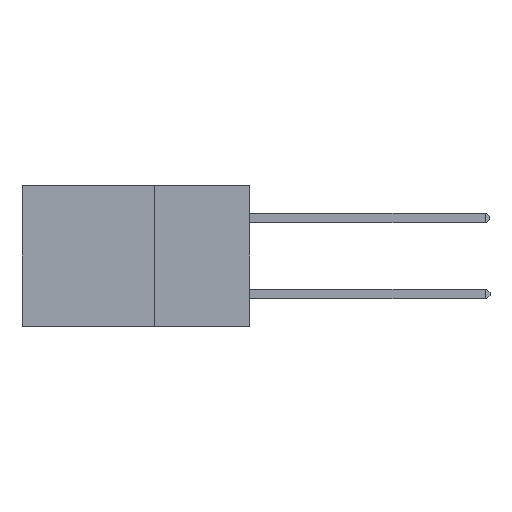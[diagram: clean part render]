
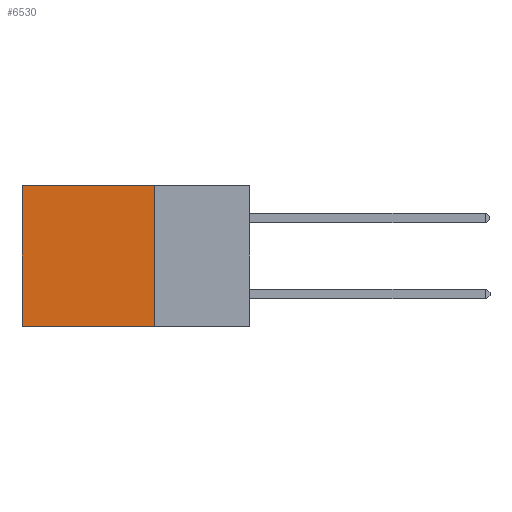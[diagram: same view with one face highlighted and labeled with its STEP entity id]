
A CAD part, left-side view. The second image highlights one B-rep face of the part: STEP entity #6530.
In plain terms, the highlighted planar face has unit normal (-1, 0, 0).
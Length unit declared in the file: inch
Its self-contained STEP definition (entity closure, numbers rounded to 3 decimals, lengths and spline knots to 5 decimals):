
#304 = AXIS2_PLACEMENT_3D ( 'NONE', #11808, #3369, #13177 ) ;
#1356 = EDGE_CURVE ( 'NONE', #13625, #13958, #12016, .T. ) ;
#2457 = CARTESIAN_POINT ( 'NONE',  ( 0.2875, 0.6, 0. ) ) ;
#3369 = DIRECTION ( 'NONE',  ( 1., 0., 0. ) ) ;
#3819 = EDGE_CURVE ( 'NONE', #12779, #13625, #6943, .T. ) ;
#3874 = EDGE_CURVE ( 'NONE', #12779, #17033, #13856, .T. ) ;
#5580 = EDGE_CURVE ( 'NONE', #17033, #13958, #14398, .T. ) ;
#6530 = ADVANCED_FACE ( 'NONE', ( #17355 ), #17137, .F. ) ;
#6943 = LINE ( 'NONE', #14657, #17375 ) ;
#7065 = VECTOR ( 'NONE', #17627, 39.37008 ) ;
#8341 = VECTOR ( 'NONE', #17480, 39.37008 ) ;
#11509 = EDGE_LOOP ( 'NONE', ( #13700, #13780, #13813, #13905 ) ) ;
#11808 = CARTESIAN_POINT ( 'NONE',  ( 0.2875, 0.25, 0. ) ) ;
#12016 = LINE ( 'NONE', #17886, #8341 ) ;
#12779 = VERTEX_POINT ( 'NONE', #16574 ) ;
#13177 = DIRECTION ( 'NONE',  ( 0., 0., -1. ) ) ;
#13539 = CARTESIAN_POINT ( 'NONE',  ( 0.2875, 0.6, 0. ) ) ;
#13625 = VERTEX_POINT ( 'NONE', #15833 ) ;
#13700 = ORIENTED_EDGE ( 'NONE', *, *, #5580, .T. ) ;
#13766 = DIRECTION ( 'NONE',  ( 0., 1., 0. ) ) ;
#13780 = ORIENTED_EDGE ( 'NONE', *, *, #1356, .F. ) ;
#13813 = ORIENTED_EDGE ( 'NONE', *, *, #3819, .F. ) ;
#13856 = LINE ( 'NONE', #13875, #16576 ) ;
#13875 = CARTESIAN_POINT ( 'NONE',  ( 0.2875, 0.25, 0. ) ) ;
#13905 = ORIENTED_EDGE ( 'NONE', *, *, #3874, .T. ) ;
#13958 = VERTEX_POINT ( 'NONE', #15017 ) ;
#14398 = LINE ( 'NONE', #2457, #7065 ) ;
#14534 = DIRECTION ( 'NONE',  ( 0., 0., -1. ) ) ;
#14657 = CARTESIAN_POINT ( 'NONE',  ( 0.2875, 0.25, 0. ) ) ;
#15017 = CARTESIAN_POINT ( 'NONE',  ( 0.2875, 0.6, -0.37 ) ) ;
#15833 = CARTESIAN_POINT ( 'NONE',  ( 0.2875, 0.25, -0.37 ) ) ;
#16574 = CARTESIAN_POINT ( 'NONE',  ( 0.2875, 0.25, 0. ) ) ;
#16576 = VECTOR ( 'NONE', #13766, 39.37008 ) ;
#17033 = VERTEX_POINT ( 'NONE', #13539 ) ;
#17137 = PLANE ( 'NONE',  #304 ) ;
#17355 = FACE_OUTER_BOUND ( 'NONE', #11509, .T. ) ;
#17375 = VECTOR ( 'NONE', #14534, 39.37008 ) ;
#17480 = DIRECTION ( 'NONE',  ( 0., 1., 0. ) ) ;
#17627 = DIRECTION ( 'NONE',  ( 0., 0., -1. ) ) ;
#17886 = CARTESIAN_POINT ( 'NONE',  ( 0.2875, 0.25, -0.37 ) ) ;
